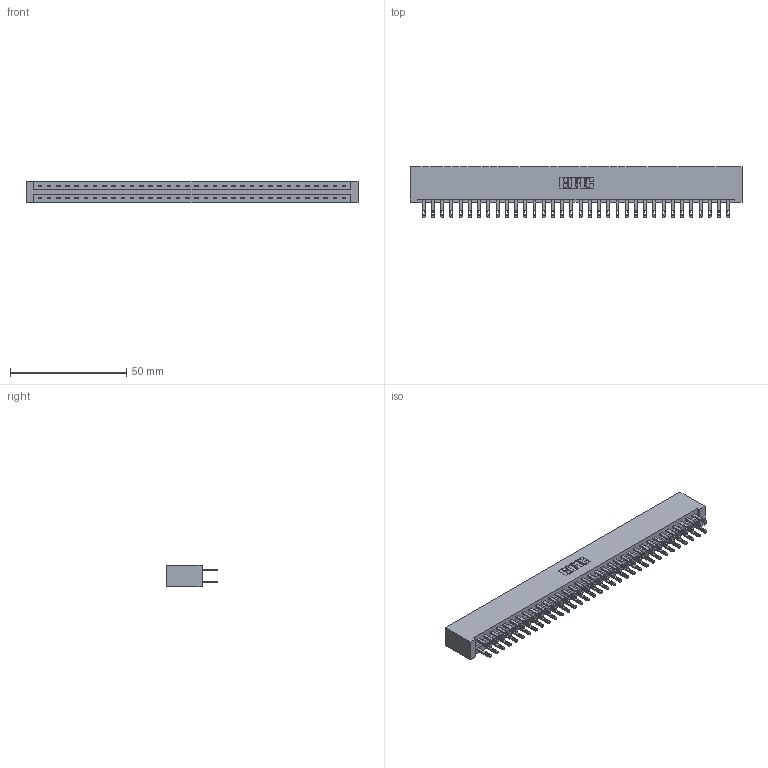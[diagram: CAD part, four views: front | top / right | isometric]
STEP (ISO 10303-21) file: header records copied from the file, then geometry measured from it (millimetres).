
FILE_DESCRIPTION (( 'STEP AP203' ), '1' );
FILE_NAME ('887-068-500-201.STEP', '2020-09-21T02:54:47', ( '' ), ( '' ), 'SwSTEP 2.0', 'SolidWorks 2020', '' );
FILE_SCHEMA (( 'CONFIG_CONTROL_DESIGN' ));
Length unit declared in the file: inch
Products named in the file (3): 887-068-500-201; 345-292-001_345-293-100; 837 Part_No Mounting Lugs
Assembly tree (69 placements, depth 2):
  887-068-500-201
    837 Part_No Mounting Lugs
    345-292-001_345-293-100  x68
Bounding box: 142.6 x 21.85 x 9.4 mm (x, y, z)
Volume: 15889.9 mm3; surface area: 18696.5 mm2
Topology: 69 solids, 69 shells, 3506 faces, 10691 edges, 7126 vertices
Faces by surface type: plane 2242, cylinder 1264
Entity records: 27049 total; most frequent: CARTESIAN_POINT 4562, ORIENTED_EDGE 4498, DIRECTION 3889, EDGE_CURVE 2249, LINE 2125, VECTOR 2125, VERTEX_POINT 1498, AXIS2_PLACEMENT_3D 882
